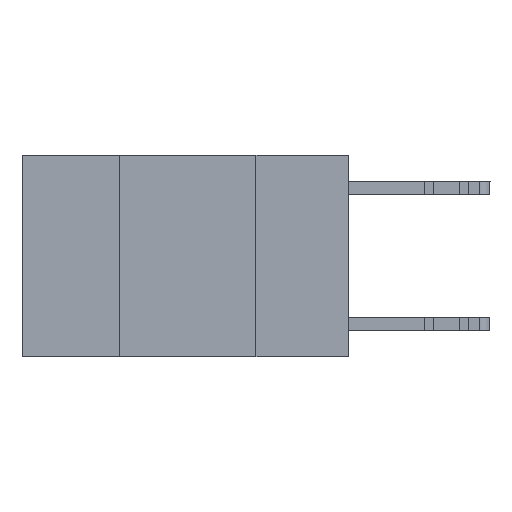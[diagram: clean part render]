
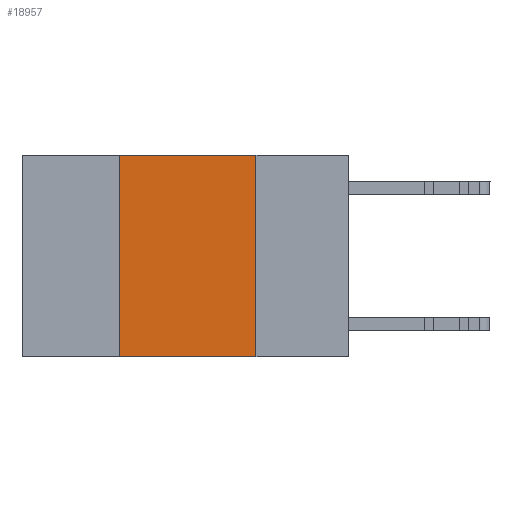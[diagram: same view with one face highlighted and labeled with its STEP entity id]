
A CAD part, left-side view. The second image highlights one B-rep face of the part: STEP entity #18957.
In plain terms, the highlighted planar face has unit normal (-1, 0, 0).
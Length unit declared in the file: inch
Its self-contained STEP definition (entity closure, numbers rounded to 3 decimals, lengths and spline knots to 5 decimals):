
#965 = ORIENTED_EDGE ( 'NONE', *, *, #17189, .F. ) ;
#4489 = DIRECTION ( 'NONE',  ( 1., 0., 0. ) ) ;
#4905 = EDGE_CURVE ( 'NONE', #5171, #17354, #11706, .T. ) ;
#5171 = VERTEX_POINT ( 'NONE', #30099 ) ;
#5324 = LINE ( 'NONE', #22237, #26246 ) ;
#6172 = AXIS2_PLACEMENT_3D ( 'NONE', #19201, #4489, #14302 ) ;
#6998 = VERTEX_POINT ( 'NONE', #30913 ) ;
#7460 = ORIENTED_EDGE ( 'NONE', *, *, #11698, .F. ) ;
#10229 = DIRECTION ( 'NONE',  ( 0., 0., -1. ) ) ;
#11637 = DIRECTION ( 'NONE',  ( 0., -1., 0. ) ) ;
#11698 = EDGE_CURVE ( 'NONE', #5171, #6998, #18595, .T. ) ;
#11706 = LINE ( 'NONE', #16779, #29989 ) ;
#11829 = EDGE_LOOP ( 'NONE', ( #13198, #965, #7460, #17786 ) ) ;
#11922 = PLANE ( 'NONE',  #6172 ) ;
#12117 = CARTESIAN_POINT ( 'NONE',  ( 0., 0.6, 0. ) ) ;
#13198 = ORIENTED_EDGE ( 'NONE', *, *, #18643, .F. ) ;
#14297 = CARTESIAN_POINT ( 'NONE',  ( 0., 0.17, 0. ) ) ;
#14302 = DIRECTION ( 'NONE',  ( 0., 0., -1. ) ) ;
#16383 = FACE_OUTER_BOUND ( 'NONE', #11829, .T. ) ;
#16590 = VECTOR ( 'NONE', #11637, 39.37008 ) ;
#16779 = CARTESIAN_POINT ( 'NONE',  ( 0., 0.6, -0.37 ) ) ;
#17189 = EDGE_CURVE ( 'NONE', #6998, #22970, #26552, .T. ) ;
#17354 = VERTEX_POINT ( 'NONE', #20006 ) ;
#17786 = ORIENTED_EDGE ( 'NONE', *, *, #4905, .T. ) ;
#18595 = LINE ( 'NONE', #28297, #28730 ) ;
#18643 = EDGE_CURVE ( 'NONE', #22970, #17354, #5324, .T. ) ;
#18957 = ADVANCED_FACE ( 'NONE', ( #16383 ), #11922, .F. ) ;
#19201 = CARTESIAN_POINT ( 'NONE',  ( 0., 0.6, 0. ) ) ;
#20006 = CARTESIAN_POINT ( 'NONE',  ( 0., 0.17, -0.37 ) ) ;
#22237 = CARTESIAN_POINT ( 'NONE',  ( 0., 0.17, 0. ) ) ;
#22970 = VERTEX_POINT ( 'NONE', #14297 ) ;
#26246 = VECTOR ( 'NONE', #10229, 39.37008 ) ;
#26460 = DIRECTION ( 'NONE',  ( 0., -1., 0. ) ) ;
#26552 = LINE ( 'NONE', #12117, #16590 ) ;
#28297 = CARTESIAN_POINT ( 'NONE',  ( 0., 0.42, 0. ) ) ;
#28730 = VECTOR ( 'NONE', #30867, 39.37008 ) ;
#29989 = VECTOR ( 'NONE', #26460, 39.37008 ) ;
#30099 = CARTESIAN_POINT ( 'NONE',  ( 0., 0.42, -0.37 ) ) ;
#30867 = DIRECTION ( 'NONE',  ( 0., 0., 1. ) ) ;
#30913 = CARTESIAN_POINT ( 'NONE',  ( 0., 0.42, 0. ) ) ;
